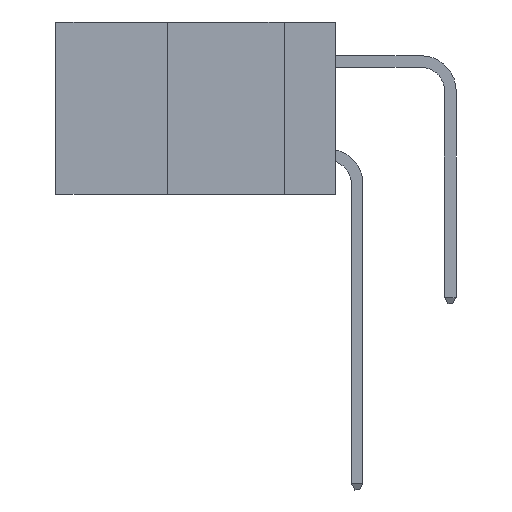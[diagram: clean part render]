
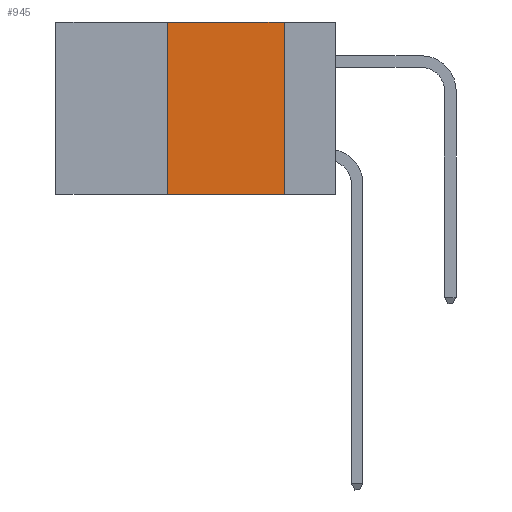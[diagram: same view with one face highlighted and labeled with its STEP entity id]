
A CAD part, left-side view. The second image highlights one B-rep face of the part: STEP entity #945.
In plain terms, the highlighted planar face has unit normal (-1, 0, 0).
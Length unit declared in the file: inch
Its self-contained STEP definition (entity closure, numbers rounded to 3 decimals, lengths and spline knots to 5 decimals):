
#498 = CARTESIAN_POINT ( 'NONE',  ( 0., 0.36, 0. ) ) ;
#738 = EDGE_CURVE ( 'NONE', #6266, #12791, #2636, .T. ) ;
#945 = ADVANCED_FACE ( 'NONE', ( #10052 ), #12177, .F. ) ;
#1064 = ORIENTED_EDGE ( 'NONE', *, *, #738, .F. ) ;
#1230 = DIRECTION ( 'NONE',  ( 0., -1., 0. ) ) ;
#2145 = DIRECTION ( 'NONE',  ( 0., 0., 1. ) ) ;
#2636 = LINE ( 'NONE', #16413, #9072 ) ;
#2907 = EDGE_CURVE ( 'NONE', #12331, #6266, #6485, .T. ) ;
#3030 = CARTESIAN_POINT ( 'NONE',  ( 0., 0.11, 0. ) ) ;
#3725 = EDGE_LOOP ( 'NONE', ( #1064, #9468, #16694, #12583 ) ) ;
#4069 = CARTESIAN_POINT ( 'NONE',  ( 0., 0.11, -0.37 ) ) ;
#5370 = CARTESIAN_POINT ( 'NONE',  ( 0., 0.6, 0. ) ) ;
#6013 = VECTOR ( 'NONE', #6811, 39.37008 ) ;
#6266 = VERTEX_POINT ( 'NONE', #3030 ) ;
#6485 = LINE ( 'NONE', #5370, #6013 ) ;
#6811 = DIRECTION ( 'NONE',  ( 0., -1., 0. ) ) ;
#7489 = EDGE_CURVE ( 'NONE', #13380, #12331, #17804, .T. ) ;
#7720 = DIRECTION ( 'NONE',  ( 1., 0., 0. ) ) ;
#8476 = CARTESIAN_POINT ( 'NONE',  ( 0., 0.6, -0.37 ) ) ;
#9072 = VECTOR ( 'NONE', #12045, 39.37008 ) ;
#9468 = ORIENTED_EDGE ( 'NONE', *, *, #2907, .F. ) ;
#10052 = FACE_OUTER_BOUND ( 'NONE', #3725, .T. ) ;
#11304 = VECTOR ( 'NONE', #1230, 39.37008 ) ;
#11335 = VECTOR ( 'NONE', #2145, 39.37008 ) ;
#12045 = DIRECTION ( 'NONE',  ( 0., 0., -1. ) ) ;
#12177 = PLANE ( 'NONE',  #16246 ) ;
#12231 = CARTESIAN_POINT ( 'NONE',  ( 0., 0.6, 0. ) ) ;
#12331 = VERTEX_POINT ( 'NONE', #15238 ) ;
#12583 = ORIENTED_EDGE ( 'NONE', *, *, #15259, .T. ) ;
#12791 = VERTEX_POINT ( 'NONE', #4069 ) ;
#13380 = VERTEX_POINT ( 'NONE', #18406 ) ;
#15238 = CARTESIAN_POINT ( 'NONE',  ( 0., 0.36, 0. ) ) ;
#15257 = LINE ( 'NONE', #8476, #11304 ) ;
#15259 = EDGE_CURVE ( 'NONE', #13380, #12791, #15257, .T. ) ;
#16246 = AXIS2_PLACEMENT_3D ( 'NONE', #12231, #7720, #16724 ) ;
#16413 = CARTESIAN_POINT ( 'NONE',  ( 0., 0.11, 0. ) ) ;
#16694 = ORIENTED_EDGE ( 'NONE', *, *, #7489, .F. ) ;
#16724 = DIRECTION ( 'NONE',  ( 0., 0., -1. ) ) ;
#17804 = LINE ( 'NONE', #498, #11335 ) ;
#18406 = CARTESIAN_POINT ( 'NONE',  ( 0., 0.36, -0.37 ) ) ;
